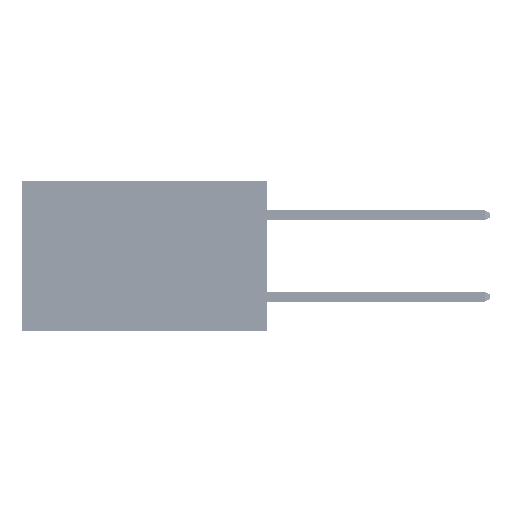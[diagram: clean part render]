
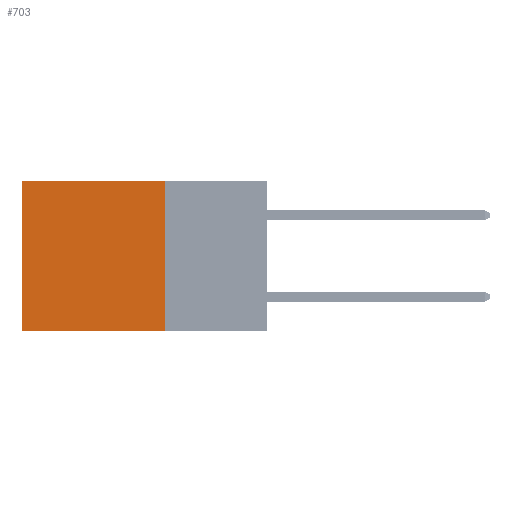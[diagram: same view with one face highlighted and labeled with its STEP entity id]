
A CAD part, left-side view. The second image highlights one B-rep face of the part: STEP entity #703.
In plain terms, the highlighted planar face has unit normal (-1, 0, 0).
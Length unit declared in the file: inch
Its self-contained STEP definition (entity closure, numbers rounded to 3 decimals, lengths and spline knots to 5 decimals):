
#703 = ADVANCED_FACE ( 'NONE', ( #10254 ), #18104, .F. ) ;
#860 = VERTEX_POINT ( 'NONE', #15012 ) ;
#867 = VECTOR ( 'NONE', #27054, 39.37008 ) ;
#1321 = LINE ( 'NONE', #23017, #44915 ) ;
#3582 = CARTESIAN_POINT ( 'NONE',  ( 0.2875, 0.25, 0. ) ) ;
#5225 = ORIENTED_EDGE ( 'NONE', *, *, #19652, .F. ) ;
#5527 = ORIENTED_EDGE ( 'NONE', *, *, #29271, .T. ) ;
#7214 = VERTEX_POINT ( 'NONE', #11648 ) ;
#10254 = FACE_OUTER_BOUND ( 'NONE', #43464, .T. ) ;
#11648 = CARTESIAN_POINT ( 'NONE',  ( 0.2875, 0.25, -0.37 ) ) ;
#12284 = CARTESIAN_POINT ( 'NONE',  ( 0.2875, 0.25, 0. ) ) ;
#12348 = DIRECTION ( 'NONE',  ( 0., 0., -1. ) ) ;
#15012 = CARTESIAN_POINT ( 'NONE',  ( 0.2875, 0.6, -0.37 ) ) ;
#15369 = DIRECTION ( 'NONE',  ( 0., 1., 0. ) ) ;
#15481 = EDGE_CURVE ( 'NONE', #22954, #7214, #1321, .T. ) ;
#18104 = PLANE ( 'NONE',  #18247 ) ;
#18247 = AXIS2_PLACEMENT_3D ( 'NONE', #3582, #21215, #39360 ) ;
#18712 = CARTESIAN_POINT ( 'NONE',  ( 0.2875, 0.25, -0.37 ) ) ;
#19652 = EDGE_CURVE ( 'NONE', #7214, #860, #43515, .T. ) ;
#21215 = DIRECTION ( 'NONE',  ( 1., 0., 0. ) ) ;
#22954 = VERTEX_POINT ( 'NONE', #26105 ) ;
#23007 = VECTOR ( 'NONE', #15369, 39.37008 ) ;
#23017 = CARTESIAN_POINT ( 'NONE',  ( 0.2875, 0.25, 0. ) ) ;
#23064 = LINE ( 'NONE', #37646, #29253 ) ;
#23470 = LINE ( 'NONE', #12284, #867 ) ;
#25722 = ORIENTED_EDGE ( 'NONE', *, *, #44514, .T. ) ;
#26105 = CARTESIAN_POINT ( 'NONE',  ( 0.2875, 0.25, 0. ) ) ;
#26369 = DIRECTION ( 'NONE',  ( 0., 0., -1. ) ) ;
#27054 = DIRECTION ( 'NONE',  ( 0., 1., 0. ) ) ;
#29253 = VECTOR ( 'NONE', #12348, 39.37008 ) ;
#29271 = EDGE_CURVE ( 'NONE', #22954, #43231, #23470, .T. ) ;
#37646 = CARTESIAN_POINT ( 'NONE',  ( 0.2875, 0.6, 0. ) ) ;
#39050 = CARTESIAN_POINT ( 'NONE',  ( 0.2875, 0.6, 0. ) ) ;
#39360 = DIRECTION ( 'NONE',  ( 0., 0., -1. ) ) ;
#43012 = ORIENTED_EDGE ( 'NONE', *, *, #15481, .F. ) ;
#43231 = VERTEX_POINT ( 'NONE', #39050 ) ;
#43464 = EDGE_LOOP ( 'NONE', ( #25722, #5225, #43012, #5527 ) ) ;
#43515 = LINE ( 'NONE', #18712, #23007 ) ;
#44514 = EDGE_CURVE ( 'NONE', #43231, #860, #23064, .T. ) ;
#44915 = VECTOR ( 'NONE', #26369, 39.37008 ) ;
